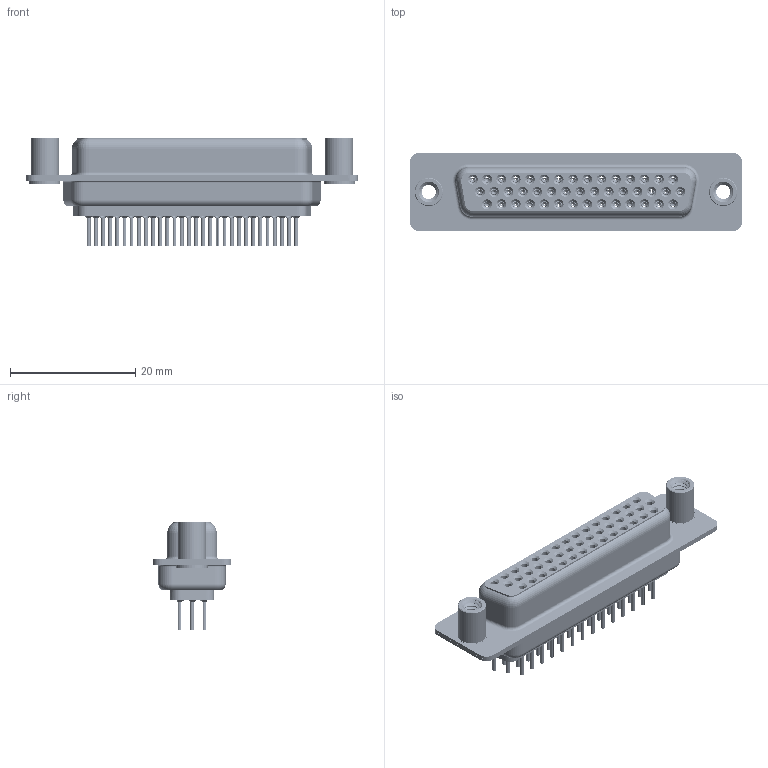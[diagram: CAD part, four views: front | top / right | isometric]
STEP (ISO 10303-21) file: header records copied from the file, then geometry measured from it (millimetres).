
FILE_DESCRIPTION (( 'STEP AP203' ), '1' );
FILE_NAME ('638-044-230-048.STEP', '2020-07-18T22:02:15', ( '' ), ( '' ), 'SwSTEP 2.0', 'SolidWorks 2020', '' );
FILE_SCHEMA (( 'CONFIG_CONTROL_DESIGN' ));
Length unit declared in the file: millimetre
Products named in the file (8): 638 Contact Row 3_30; 638 Shell Front_44 Contacts; 638-044-230-048; 638 Shell Rear_44 Contacts; 638 Contact Row 2_30; 638 4-40 Threaded Standoff; 638 Housing_44 Contacts; 638 Contact Row 1_30
Assembly tree (49 placements, depth 2):
  638-044-230-048
    638 Housing_44 Contacts
    638 Shell Front_44 Contacts
    638 Shell Rear_44 Contacts
    638 Contact Row 1_30  x15
    638 Contact Row 2_30  x15
    638 Contact Row 3_30  x14
    638 4-40 Threaded Standoff  x2
Bounding box: 53.04 x 12.6 x 17.3 mm (x, y, z)
Volume: 3326.4 mm3; surface area: 12944.6 mm2
Topology: 49 solids, 49 shells, 5901 faces, 15033 edges, 9331 vertices
Faces by surface type: cylinder 1617, plane 1433, torus 1201, bspline 886, cone 764
Entity records: 40631 total; most frequent: CARTESIAN_POINT 11214, DIRECTION 6072, ORIENTED_EDGE 5510, EDGE_CURVE 2755, AXIS2_PLACEMENT_3D 2555, VERTEX_POINT 1740, EDGE_LOOP 1415, CIRCLE 1395
